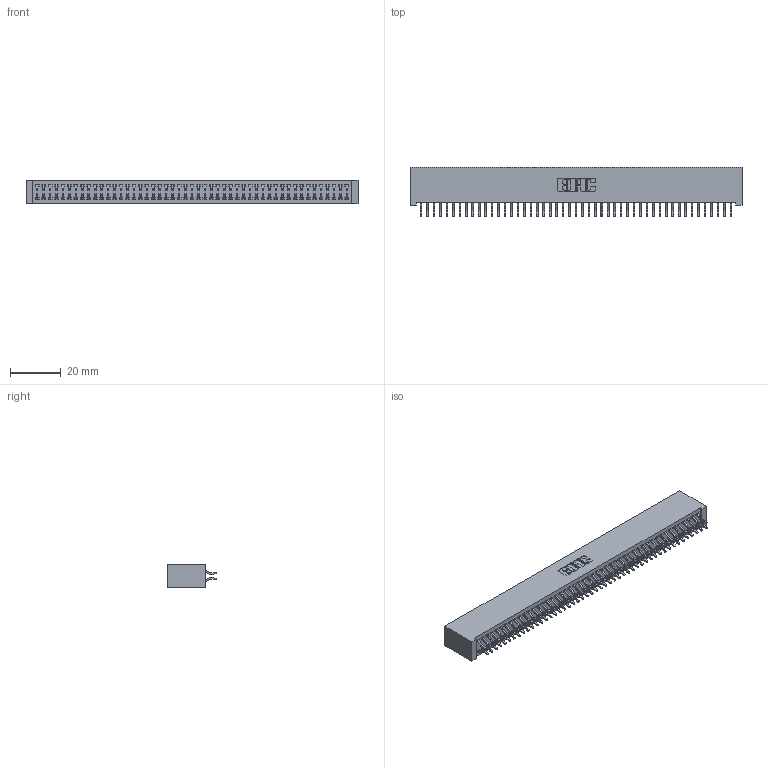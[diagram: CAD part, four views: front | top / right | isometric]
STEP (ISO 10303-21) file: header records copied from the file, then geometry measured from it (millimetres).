
FILE_DESCRIPTION (( 'STEP AP203' ), '1' );
FILE_NAME ('392-098-556-201.STEP', '2019-10-09T20:30:53', ( '' ), ( '' ), 'SwSTEP 2.0', 'SolidWorks 2016', '' );
FILE_SCHEMA (( 'CONFIG_CONTROL_DESIGN' ));
Length unit declared in the file: inch
Products named in the file (3): 342 Part_Lugless; 345-292-001_556 Tail; 392-098-556-201
Assembly tree (99 placements, depth 2):
  392-098-556-201
    342 Part_Lugless
    345-292-001_556 Tail  x98
Bounding box: 130.71 x 19.58 x 9.4 mm (x, y, z)
Volume: 12214.3 mm3; surface area: 20405.5 mm2
Topology: 99 solids, 99 shells, 5786 faces, 17229 edges, 11354 vertices
Faces by surface type: plane 3982, cylinder 1804
Entity records: 30429 total; most frequent: CARTESIAN_POINT 5046, ORIENTED_EDGE 4970, DIRECTION 4281, EDGE_CURVE 2485, VECTOR 2357, LINE 2357, VERTEX_POINT 1654, AXIS2_PLACEMENT_3D 962
